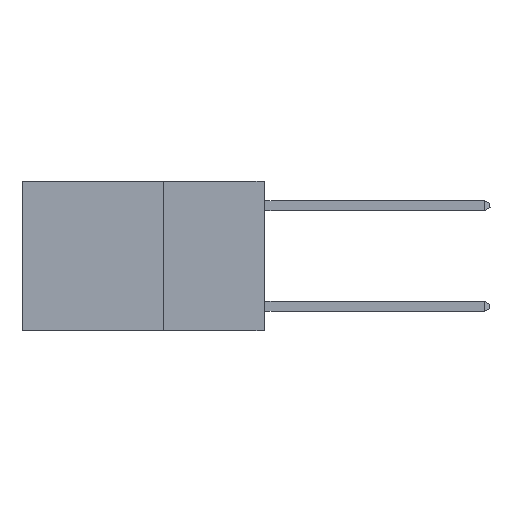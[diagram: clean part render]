
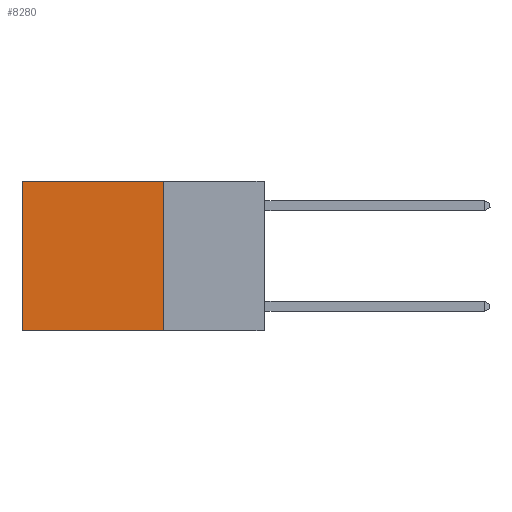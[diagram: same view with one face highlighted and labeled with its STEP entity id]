
A CAD part, left-side view. The second image highlights one B-rep face of the part: STEP entity #8280.
In plain terms, the highlighted planar face has unit normal (-1, 0, 0).
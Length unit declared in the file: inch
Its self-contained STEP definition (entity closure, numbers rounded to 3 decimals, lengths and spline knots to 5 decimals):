
#290 = EDGE_CURVE ( 'NONE', #1888, #10914, #4116, .T. ) ;
#456 = ORIENTED_EDGE ( 'NONE', *, *, #2795, .T. ) ;
#892 = CARTESIAN_POINT ( 'NONE',  ( 0.2625, 0.25, 0. ) ) ;
#1722 = VECTOR ( 'NONE', #10313, 39.37008 ) ;
#1810 = CARTESIAN_POINT ( 'NONE',  ( 0.2625, 0.25, -0.37 ) ) ;
#1888 = VERTEX_POINT ( 'NONE', #6074 ) ;
#2671 = ORIENTED_EDGE ( 'NONE', *, *, #290, .T. ) ;
#2795 = EDGE_CURVE ( 'NONE', #10914, #10037, #11702, .T. ) ;
#2833 = VERTEX_POINT ( 'NONE', #1810 ) ;
#3033 = DIRECTION ( 'NONE',  ( 0., 0., -1. ) ) ;
#3303 = CARTESIAN_POINT ( 'NONE',  ( 0.2625, 0.6, 0. ) ) ;
#3576 = CARTESIAN_POINT ( 'NONE',  ( 0.2625, 0.25, -0.37 ) ) ;
#3829 = FACE_OUTER_BOUND ( 'NONE', #8776, .T. ) ;
#4116 = LINE ( 'NONE', #6041, #7611 ) ;
#5024 = VECTOR ( 'NONE', #12296, 39.37008 ) ;
#5033 = ORIENTED_EDGE ( 'NONE', *, *, #11539, .F. ) ;
#5750 = CARTESIAN_POINT ( 'NONE',  ( 0.2625, 0.25, 0. ) ) ;
#6033 = CARTESIAN_POINT ( 'NONE',  ( 0.2625, 0.6, -0.37 ) ) ;
#6041 = CARTESIAN_POINT ( 'NONE',  ( 0.2625, 0.25, 0. ) ) ;
#6074 = CARTESIAN_POINT ( 'NONE',  ( 0.2625, 0.25, 0. ) ) ;
#7075 = CARTESIAN_POINT ( 'NONE',  ( 0.2625, 0.6, 0. ) ) ;
#7227 = LINE ( 'NONE', #3576, #1722 ) ;
#7611 = VECTOR ( 'NONE', #9858, 39.37008 ) ;
#7630 = ORIENTED_EDGE ( 'NONE', *, *, #9865, .F. ) ;
#8280 = ADVANCED_FACE ( 'NONE', ( #3829 ), #9501, .F. ) ;
#8667 = DIRECTION ( 'NONE',  ( 1., 0., 0. ) ) ;
#8776 = EDGE_LOOP ( 'NONE', ( #456, #7630, #5033, #2671 ) ) ;
#9501 = PLANE ( 'NONE',  #9630 ) ;
#9630 = AXIS2_PLACEMENT_3D ( 'NONE', #5750, #8667, #3033 ) ;
#9858 = DIRECTION ( 'NONE',  ( 0., 1., 0. ) ) ;
#9865 = EDGE_CURVE ( 'NONE', #2833, #10037, #7227, .T. ) ;
#10037 = VERTEX_POINT ( 'NONE', #6033 ) ;
#10313 = DIRECTION ( 'NONE',  ( 0., 1., 0. ) ) ;
#10383 = LINE ( 'NONE', #892, #5024 ) ;
#10914 = VERTEX_POINT ( 'NONE', #3303 ) ;
#11335 = VECTOR ( 'NONE', #11762, 39.37008 ) ;
#11539 = EDGE_CURVE ( 'NONE', #1888, #2833, #10383, .T. ) ;
#11702 = LINE ( 'NONE', #7075, #11335 ) ;
#11762 = DIRECTION ( 'NONE',  ( 0., 0., -1. ) ) ;
#12296 = DIRECTION ( 'NONE',  ( 0., 0., -1. ) ) ;
